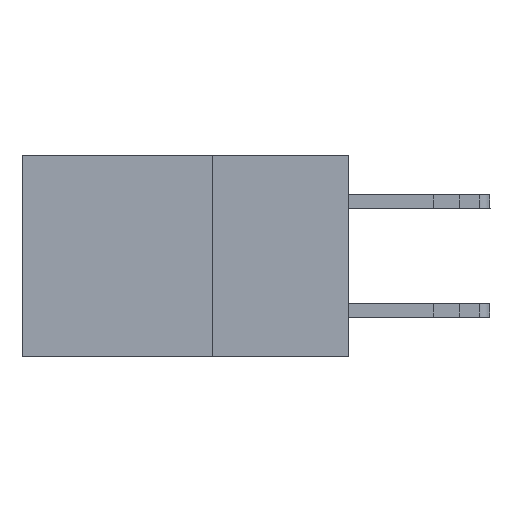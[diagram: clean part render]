
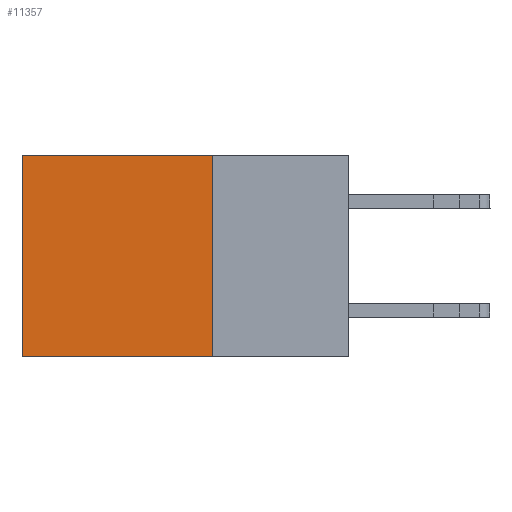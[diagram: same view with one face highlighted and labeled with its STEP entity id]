
A CAD part, left-side view. The second image highlights one B-rep face of the part: STEP entity #11357.
In plain terms, the highlighted planar face has unit normal (-1, 0, 0).
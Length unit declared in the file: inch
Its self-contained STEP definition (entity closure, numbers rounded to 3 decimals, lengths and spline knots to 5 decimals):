
#622 = VERTEX_POINT ( 'NONE', #3030 ) ;
#833 = ORIENTED_EDGE ( 'NONE', *, *, #4224, .F. ) ;
#890 = VERTEX_POINT ( 'NONE', #1084 ) ;
#1084 = CARTESIAN_POINT ( 'NONE',  ( 0.2615, 0.6, -0.37 ) ) ;
#2429 = AXIS2_PLACEMENT_3D ( 'NONE', #3346, #4295, #8857 ) ;
#2630 = LINE ( 'NONE', #7201, #5062 ) ;
#2648 = CARTESIAN_POINT ( 'NONE',  ( 0.2615, 0.25, -0.37 ) ) ;
#3023 = EDGE_CURVE ( 'NONE', #622, #10263, #8971, .T. ) ;
#3030 = CARTESIAN_POINT ( 'NONE',  ( 0.2615, 0.25, 0. ) ) ;
#3290 = PLANE ( 'NONE',  #2429 ) ;
#3346 = CARTESIAN_POINT ( 'NONE',  ( 0.2615, 0.25, -0.37 ) ) ;
#3513 = DIRECTION ( 'NONE',  ( 0., 0., -1. ) ) ;
#4224 = EDGE_CURVE ( 'NONE', #10263, #890, #10492, .T. ) ;
#4293 = CARTESIAN_POINT ( 'NONE',  ( 0.2615, 0.25, -0.37 ) ) ;
#4295 = DIRECTION ( 'NONE',  ( 1., 0., 0. ) ) ;
#4347 = FACE_OUTER_BOUND ( 'NONE', #5147, .T. ) ;
#5062 = VECTOR ( 'NONE', #8894, 39.37008 ) ;
#5113 = DIRECTION ( 'NONE',  ( 0., 1., 0. ) ) ;
#5147 = EDGE_LOOP ( 'NONE', ( #9990, #833, #9208, #5922 ) ) ;
#5922 = ORIENTED_EDGE ( 'NONE', *, *, #7331, .T. ) ;
#6489 = CARTESIAN_POINT ( 'NONE',  ( 0.2615, 0.25, 0. ) ) ;
#7116 = EDGE_CURVE ( 'NONE', #11131, #890, #2630, .T. ) ;
#7201 = CARTESIAN_POINT ( 'NONE',  ( 0.2615, 0.6, -0.37 ) ) ;
#7331 = EDGE_CURVE ( 'NONE', #622, #11131, #8328, .T. ) ;
#8305 = CARTESIAN_POINT ( 'NONE',  ( 0.2615, 0.6, 0. ) ) ;
#8328 = LINE ( 'NONE', #6489, #11054 ) ;
#8857 = DIRECTION ( 'NONE',  ( 0., 0., -1. ) ) ;
#8894 = DIRECTION ( 'NONE',  ( 0., 0., -1. ) ) ;
#8971 = LINE ( 'NONE', #2648, #10526 ) ;
#9208 = ORIENTED_EDGE ( 'NONE', *, *, #3023, .F. ) ;
#9763 = VECTOR ( 'NONE', #5113, 39.37008 ) ;
#9990 = ORIENTED_EDGE ( 'NONE', *, *, #7116, .T. ) ;
#10060 = DIRECTION ( 'NONE',  ( 0., 1., 0. ) ) ;
#10263 = VERTEX_POINT ( 'NONE', #10822 ) ;
#10492 = LINE ( 'NONE', #4293, #9763 ) ;
#10526 = VECTOR ( 'NONE', #3513, 39.37008 ) ;
#10822 = CARTESIAN_POINT ( 'NONE',  ( 0.2615, 0.25, -0.37 ) ) ;
#11054 = VECTOR ( 'NONE', #10060, 39.37008 ) ;
#11131 = VERTEX_POINT ( 'NONE', #8305 ) ;
#11357 = ADVANCED_FACE ( 'NONE', ( #4347 ), #3290, .F. ) ;
